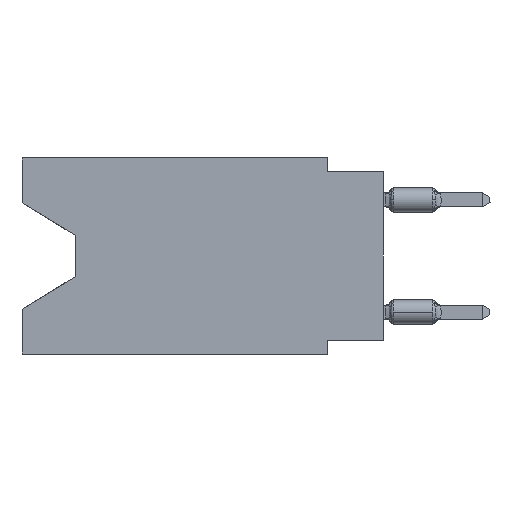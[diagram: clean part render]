
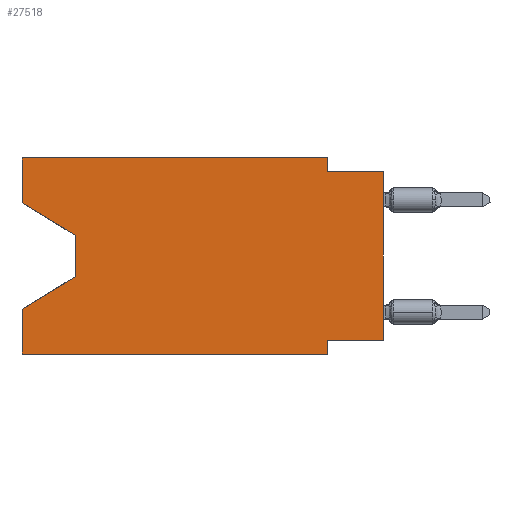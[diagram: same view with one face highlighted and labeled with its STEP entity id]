
A CAD part, left-side view. The second image highlights one B-rep face of the part: STEP entity #27518.
In plain terms, the highlighted planar face has unit normal (-1, 0, 0).
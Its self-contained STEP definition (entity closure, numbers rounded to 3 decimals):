
#227 = CARTESIAN_POINT ( 'NONE',  ( 0., 16.383, 0. ) ) ;
#780 = LINE ( 'NONE', #26759, #3013 ) ;
#1932 = VERTEX_POINT ( 'NONE', #34352 ) ;
#2072 = EDGE_CURVE ( 'NONE', #25929, #16330, #19871, .T. ) ;
#2240 = ORIENTED_EDGE ( 'NONE', *, *, #2072, .T. ) ;
#2760 = CARTESIAN_POINT ( 'NONE',  ( 0., 16.383, -2.038 ) ) ;
#2943 = DIRECTION ( 'NONE',  ( 0., 1., 0. ) ) ;
#3013 = VECTOR ( 'NONE', #39735, 1000. ) ;
#3451 = VERTEX_POINT ( 'NONE', #23762 ) ;
#3781 = VERTEX_POINT ( 'NONE', #27156 ) ;
#4176 = ORIENTED_EDGE ( 'NONE', *, *, #31746, .F. ) ;
#4177 = EDGE_CURVE ( 'NONE', #13658, #3451, #6826, .T. ) ;
#4447 = VERTEX_POINT ( 'NONE', #9122 ) ;
#5471 = DIRECTION ( 'NONE',  ( 0., 0., 1. ) ) ;
#6118 = VERTEX_POINT ( 'NONE', #31650 ) ;
#6396 = CARTESIAN_POINT ( 'NONE',  ( 0., 16.383, 0. ) ) ;
#6821 = FACE_OUTER_BOUND ( 'NONE', #17023, .T. ) ;
#6826 = LINE ( 'NONE', #38391, #39072 ) ;
#7033 = DIRECTION ( 'NONE',  ( 0., 0., -1. ) ) ;
#7074 = ORIENTED_EDGE ( 'NONE', *, *, #21203, .T. ) ;
#7345 = VECTOR ( 'NONE', #5471, 1000. ) ;
#7937 = LINE ( 'NONE', #24525, #39562 ) ;
#8372 = ORIENTED_EDGE ( 'NONE', *, *, #31956, .F. ) ;
#8416 = VECTOR ( 'NONE', #13778, 1000. ) ;
#8731 = EDGE_CURVE ( 'NONE', #3781, #16330, #39333, .T. ) ;
#9122 = CARTESIAN_POINT ( 'NONE',  ( 0., 16.383, 0. ) ) ;
#9125 = LINE ( 'NONE', #19353, #12625 ) ;
#9155 = ORIENTED_EDGE ( 'NONE', *, *, #4177, .F. ) ;
#9556 = ORIENTED_EDGE ( 'NONE', *, *, #30076, .F. ) ;
#9750 = CARTESIAN_POINT ( 'NONE',  ( 0., 0., -8.255 ) ) ;
#9963 = CARTESIAN_POINT ( 'NONE',  ( 0., 2.54, -8.89 ) ) ;
#10014 = PLANE ( 'NONE',  #40428 ) ;
#12625 = VECTOR ( 'NONE', #31704, 1000. ) ;
#13658 = VERTEX_POINT ( 'NONE', #19209 ) ;
#13688 = CARTESIAN_POINT ( 'NONE',  ( 0., 16.383, -8.89 ) ) ;
#13778 = DIRECTION ( 'NONE',  ( 0., 0., -1. ) ) ;
#15306 = LINE ( 'NONE', #28295, #17576 ) ;
#16330 = VERTEX_POINT ( 'NONE', #35545 ) ;
#16525 = EDGE_CURVE ( 'NONE', #25929, #1932, #37847, .T. ) ;
#17023 = EDGE_LOOP ( 'NONE', ( #22285, #41191, #36505, #39881, #2240, #31476, #17740, #7074, #9155, #4176, #9556, #8372 ) ) ;
#17576 = VECTOR ( 'NONE', #18691, 1000. ) ;
#17717 = DIRECTION ( 'NONE',  ( 0., 0., -1. ) ) ;
#17740 = ORIENTED_EDGE ( 'NONE', *, *, #32499, .F. ) ;
#17802 = EDGE_CURVE ( 'NONE', #32180, #6118, #19579, .T. ) ;
#18691 = DIRECTION ( 'NONE',  ( 0., 0., 1. ) ) ;
#19209 = CARTESIAN_POINT ( 'NONE',  ( 0., 2.54, -0.635 ) ) ;
#19353 = CARTESIAN_POINT ( 'NONE',  ( 0., 16.383, 0. ) ) ;
#19390 = LINE ( 'NONE', #227, #39592 ) ;
#19579 = LINE ( 'NONE', #2760, #27087 ) ;
#19871 = LINE ( 'NONE', #13688, #34237 ) ;
#20867 = CARTESIAN_POINT ( 'NONE',  ( 0., 16.383, -2.038 ) ) ;
#21203 = EDGE_CURVE ( 'NONE', #25636, #3451, #15306, .T. ) ;
#22285 = ORIENTED_EDGE ( 'NONE', *, *, #17802, .T. ) ;
#22357 = DIRECTION ( 'NONE',  ( 0., -0.855, -0.519 ) ) ;
#22913 = CARTESIAN_POINT ( 'NONE',  ( 0., 2.54, 0. ) ) ;
#23762 = CARTESIAN_POINT ( 'NONE',  ( 0., 0., -0.635 ) ) ;
#23955 = EDGE_CURVE ( 'NONE', #28140, #1932, #780, .T. ) ;
#24525 = CARTESIAN_POINT ( 'NONE',  ( 0., 13.97, -3.505 ) ) ;
#24789 = CARTESIAN_POINT ( 'NONE',  ( 0., 16.383, -8.89 ) ) ;
#24868 = CARTESIAN_POINT ( 'NONE',  ( 0., 16.383, 0. ) ) ;
#25561 = DIRECTION ( 'NONE',  ( 0., 0., 1. ) ) ;
#25636 = VERTEX_POINT ( 'NONE', #32481 ) ;
#25929 = VERTEX_POINT ( 'NONE', #24789 ) ;
#26759 = CARTESIAN_POINT ( 'NONE',  ( 0., 13.97, -5.385 ) ) ;
#27087 = VECTOR ( 'NONE', #22357, 1000. ) ;
#27156 = CARTESIAN_POINT ( 'NONE',  ( 0., 2.54, -8.255 ) ) ;
#27514 = CARTESIAN_POINT ( 'NONE',  ( 0., 2.54, 0. ) ) ;
#27518 = ADVANCED_FACE ( 'NONE', ( #6821 ), #10014, .F. ) ;
#28140 = VERTEX_POINT ( 'NONE', #34999 ) ;
#28295 = CARTESIAN_POINT ( 'NONE',  ( 0., 0., 0. ) ) ;
#28725 = VECTOR ( 'NONE', #17717, 1000. ) ;
#29889 = DIRECTION ( 'NONE',  ( 0., -1., 0. ) ) ;
#30076 = EDGE_CURVE ( 'NONE', #4447, #33079, #9125, .T. ) ;
#31450 = VECTOR ( 'NONE', #2943, 1000. ) ;
#31476 = ORIENTED_EDGE ( 'NONE', *, *, #8731, .F. ) ;
#31650 = CARTESIAN_POINT ( 'NONE',  ( 0., 13.97, -3.505 ) ) ;
#31704 = DIRECTION ( 'NONE',  ( 0., -1., 0. ) ) ;
#31746 = EDGE_CURVE ( 'NONE', #33079, #13658, #39642, .T. ) ;
#31956 = EDGE_CURVE ( 'NONE', #32180, #4447, #19390, .T. ) ;
#32112 = LINE ( 'NONE', #9750, #31450 ) ;
#32180 = VERTEX_POINT ( 'NONE', #20867 ) ;
#32481 = CARTESIAN_POINT ( 'NONE',  ( 0., 0., -8.255 ) ) ;
#32499 = EDGE_CURVE ( 'NONE', #25636, #3781, #32112, .T. ) ;
#33079 = VERTEX_POINT ( 'NONE', #22913 ) ;
#33912 = DIRECTION ( 'NONE',  ( 0., 0., -1. ) ) ;
#34237 = VECTOR ( 'NONE', #29889, 1000. ) ;
#34352 = CARTESIAN_POINT ( 'NONE',  ( 0., 16.383, -6.852 ) ) ;
#34999 = CARTESIAN_POINT ( 'NONE',  ( 0., 13.97, -5.385 ) ) ;
#35214 = DIRECTION ( 'NONE',  ( 0., -1., 0. ) ) ;
#35545 = CARTESIAN_POINT ( 'NONE',  ( 0., 2.54, -8.89 ) ) ;
#36505 = ORIENTED_EDGE ( 'NONE', *, *, #23955, .T. ) ;
#37847 = LINE ( 'NONE', #24868, #7345 ) ;
#37867 = EDGE_CURVE ( 'NONE', #6118, #28140, #7937, .T. ) ;
#38391 = CARTESIAN_POINT ( 'NONE',  ( 0., 0., -0.635 ) ) ;
#38748 = DIRECTION ( 'NONE',  ( 1., 0., 0. ) ) ;
#39072 = VECTOR ( 'NONE', #35214, 1000. ) ;
#39333 = LINE ( 'NONE', #9963, #8416 ) ;
#39562 = VECTOR ( 'NONE', #33912, 1000. ) ;
#39592 = VECTOR ( 'NONE', #25561, 1000. ) ;
#39642 = LINE ( 'NONE', #27514, #28725 ) ;
#39735 = DIRECTION ( 'NONE',  ( 0., 0.855, -0.519 ) ) ;
#39881 = ORIENTED_EDGE ( 'NONE', *, *, #16525, .F. ) ;
#40428 = AXIS2_PLACEMENT_3D ( 'NONE', #6396, #38748, #7033 ) ;
#41191 = ORIENTED_EDGE ( 'NONE', *, *, #37867, .T. ) ;
